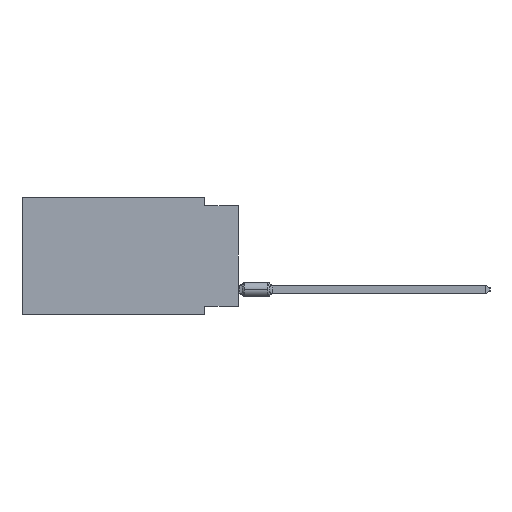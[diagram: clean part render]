
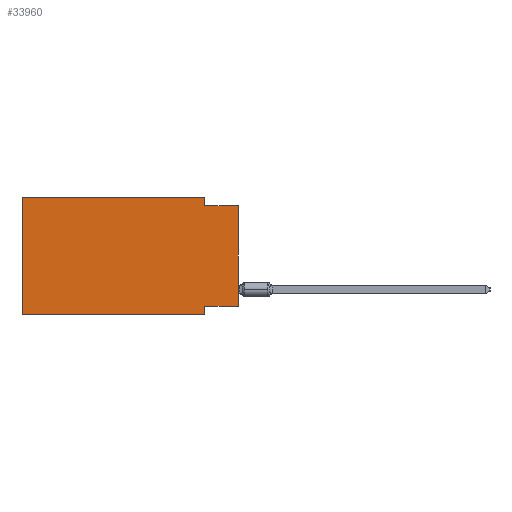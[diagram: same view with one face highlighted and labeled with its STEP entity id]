
A CAD part, left-side view. The second image highlights one B-rep face of the part: STEP entity #33960.
In plain terms, the highlighted planar face has unit normal (-1, 0, 0).
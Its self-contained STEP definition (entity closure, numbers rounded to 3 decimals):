
#666 = CARTESIAN_POINT ( 'NONE',  ( 0., 0., -0.635 ) ) ;
#1416 = ORIENTED_EDGE ( 'NONE', *, *, #74585, .F. ) ;
#5002 = LINE ( 'NONE', #17769, #57962 ) ;
#5089 = ORIENTED_EDGE ( 'NONE', *, *, #42536, .T. ) ;
#6260 = CARTESIAN_POINT ( 'NONE',  ( 0., 2.54, -8.89 ) ) ;
#6434 = CARTESIAN_POINT ( 'NONE',  ( 0., 16.383, 0. ) ) ;
#7208 = EDGE_CURVE ( 'NONE', #54480, #33156, #69091, .T. ) ;
#7264 = PLANE ( 'NONE',  #61356 ) ;
#8280 = VECTOR ( 'NONE', #14051, 1000. ) ;
#9004 = VECTOR ( 'NONE', #80080, 1000. ) ;
#10235 = CARTESIAN_POINT ( 'NONE',  ( 0., 0., -0.635 ) ) ;
#10671 = VERTEX_POINT ( 'NONE', #10235 ) ;
#11246 = EDGE_CURVE ( 'NONE', #45365, #27779, #37306, .T. ) ;
#11950 = VERTEX_POINT ( 'NONE', #37021 ) ;
#14051 = DIRECTION ( 'NONE',  ( 0., 0., 1. ) ) ;
#17769 = CARTESIAN_POINT ( 'NONE',  ( 0., 2.54, -8.89 ) ) ;
#19609 = DIRECTION ( 'NONE',  ( 0., -1., 0. ) ) ;
#21812 = VERTEX_POINT ( 'NONE', #55446 ) ;
#24085 = CARTESIAN_POINT ( 'NONE',  ( 0., 16.383, 0. ) ) ;
#24149 = CARTESIAN_POINT ( 'NONE',  ( 0., 16.383, 0. ) ) ;
#25429 = DIRECTION ( 'NONE',  ( 0., -1., 0. ) ) ;
#26619 = LINE ( 'NONE', #666, #32956 ) ;
#27779 = VERTEX_POINT ( 'NONE', #47751 ) ;
#28031 = LINE ( 'NONE', #47002, #62915 ) ;
#30132 = DIRECTION ( 'NONE',  ( 0., 1., 0. ) ) ;
#31657 = ORIENTED_EDGE ( 'NONE', *, *, #61177, .F. ) ;
#32956 = VECTOR ( 'NONE', #19609, 1000. ) ;
#33156 = VERTEX_POINT ( 'NONE', #6260 ) ;
#33653 = VERTEX_POINT ( 'NONE', #76987 ) ;
#33960 = ADVANCED_FACE ( 'NONE', ( #45609 ), #7264, .F. ) ;
#37021 = CARTESIAN_POINT ( 'NONE',  ( 0., 2.54, -0.635 ) ) ;
#37306 = LINE ( 'NONE', #24149, #58755 ) ;
#42536 = EDGE_CURVE ( 'NONE', #33653, #10671, #58974, .T. ) ;
#44804 = VECTOR ( 'NONE', #30132, 1000. ) ;
#45156 = VECTOR ( 'NONE', #25429, 1000. ) ;
#45346 = ORIENTED_EDGE ( 'NONE', *, *, #61201, .F. ) ;
#45365 = VERTEX_POINT ( 'NONE', #6434 ) ;
#45609 = FACE_OUTER_BOUND ( 'NONE', #66929, .T. ) ;
#47002 = CARTESIAN_POINT ( 'NONE',  ( 0., 2.54, 0. ) ) ;
#47751 = CARTESIAN_POINT ( 'NONE',  ( 0., 2.54, 0. ) ) ;
#48471 = DIRECTION ( 'NONE',  ( 0., -1., 0. ) ) ;
#49625 = LINE ( 'NONE', #24085, #9004 ) ;
#51374 = DIRECTION ( 'NONE',  ( 1., 0., 0. ) ) ;
#53738 = DIRECTION ( 'NONE',  ( 0., 0., -1. ) ) ;
#54480 = VERTEX_POINT ( 'NONE', #57548 ) ;
#54891 = CARTESIAN_POINT ( 'NONE',  ( 0., 0., -8.255 ) ) ;
#55446 = CARTESIAN_POINT ( 'NONE',  ( 0., 2.54, -8.255 ) ) ;
#57548 = CARTESIAN_POINT ( 'NONE',  ( 0., 16.383, -8.89 ) ) ;
#57655 = EDGE_CURVE ( 'NONE', #27779, #11950, #28031, .T. ) ;
#57962 = VECTOR ( 'NONE', #68048, 1000. ) ;
#58755 = VECTOR ( 'NONE', #48471, 1000. ) ;
#58974 = LINE ( 'NONE', #64332, #8280 ) ;
#61177 = EDGE_CURVE ( 'NONE', #33653, #21812, #75434, .T. ) ;
#61201 = EDGE_CURVE ( 'NONE', #21812, #33156, #5002, .T. ) ;
#61356 = AXIS2_PLACEMENT_3D ( 'NONE', #66082, #51374, #53738 ) ;
#62915 = VECTOR ( 'NONE', #72117, 1000. ) ;
#64332 = CARTESIAN_POINT ( 'NONE',  ( 0., 0., 0. ) ) ;
#66082 = CARTESIAN_POINT ( 'NONE',  ( 0., 16.383, 0. ) ) ;
#66929 = EDGE_LOOP ( 'NONE', ( #5089, #79102, #73558, #72431, #1416, #70143, #45346, #31657 ) ) ;
#68048 = DIRECTION ( 'NONE',  ( 0., 0., -1. ) ) ;
#69091 = LINE ( 'NONE', #69909, #45156 ) ;
#69909 = CARTESIAN_POINT ( 'NONE',  ( 0., 16.383, -8.89 ) ) ;
#70143 = ORIENTED_EDGE ( 'NONE', *, *, #7208, .T. ) ;
#72117 = DIRECTION ( 'NONE',  ( 0., 0., -1. ) ) ;
#72431 = ORIENTED_EDGE ( 'NONE', *, *, #11246, .F. ) ;
#73558 = ORIENTED_EDGE ( 'NONE', *, *, #57655, .F. ) ;
#74585 = EDGE_CURVE ( 'NONE', #54480, #45365, #49625, .T. ) ;
#75434 = LINE ( 'NONE', #54891, #44804 ) ;
#76732 = EDGE_CURVE ( 'NONE', #11950, #10671, #26619, .T. ) ;
#76987 = CARTESIAN_POINT ( 'NONE',  ( 0., 0., -8.255 ) ) ;
#79102 = ORIENTED_EDGE ( 'NONE', *, *, #76732, .F. ) ;
#80080 = DIRECTION ( 'NONE',  ( 0., 0., 1. ) ) ;
